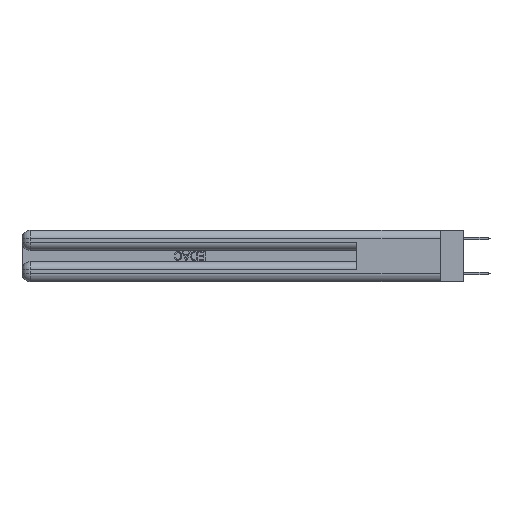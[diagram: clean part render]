
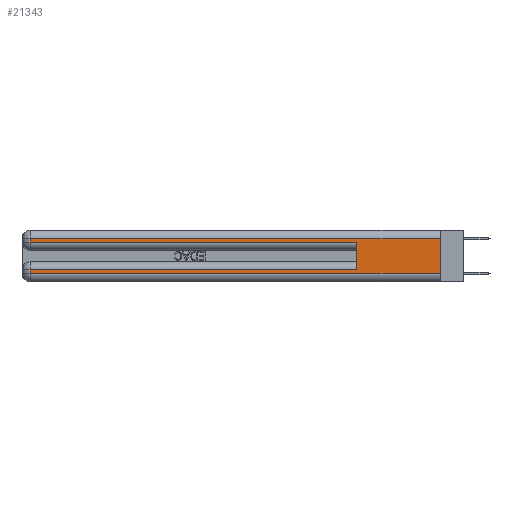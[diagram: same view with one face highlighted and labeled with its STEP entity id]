
A CAD part, left-side view. The second image highlights one B-rep face of the part: STEP entity #21343.
In plain terms, the highlighted planar face has unit normal (-1, 0, 0).
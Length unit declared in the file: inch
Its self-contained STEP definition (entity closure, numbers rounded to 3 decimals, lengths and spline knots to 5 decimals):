
#115 = CARTESIAN_POINT ( 'NONE',  ( 0., 0., 0.37 ) ) ;
#139 = VECTOR ( 'NONE', #22408, 39.37008 ) ;
#623 = ORIENTED_EDGE ( 'NONE', *, *, #24026, .T. ) ;
#768 = CARTESIAN_POINT ( 'NONE',  ( 0., 0., 0.085 ) ) ;
#996 = LINE ( 'NONE', #28972, #139 ) ;
#1272 = CARTESIAN_POINT ( 'NONE',  ( 0., 2.94, 0.31 ) ) ;
#1301 = CARTESIAN_POINT ( 'NONE',  ( 0., 0.6, 0.145 ) ) ;
#1329 = LINE ( 'NONE', #10955, #8237 ) ;
#2145 = ORIENTED_EDGE ( 'NONE', *, *, #18028, .T. ) ;
#3012 = LINE ( 'NONE', #26530, #22040 ) ;
#3297 = DIRECTION ( 'NONE',  ( 0., -1., 0. ) ) ;
#3968 = ORIENTED_EDGE ( 'NONE', *, *, #22830, .T. ) ;
#5042 = CARTESIAN_POINT ( 'NONE',  ( 0., 0., 0.31 ) ) ;
#5150 = DIRECTION ( 'NONE',  ( 1., 0., 0. ) ) ;
#6066 = VECTOR ( 'NONE', #25166, 39.37008 ) ;
#6242 = CARTESIAN_POINT ( 'NONE',  ( 0., 2.94, 0.37 ) ) ;
#6951 = ORIENTED_EDGE ( 'NONE', *, *, #24611, .F. ) ;
#7190 = VERTEX_POINT ( 'NONE', #26090 ) ;
#7719 = CARTESIAN_POINT ( 'NONE',  ( 0., 0.6, 0.285 ) ) ;
#7885 = AXIS2_PLACEMENT_3D ( 'NONE', #115, #5150, #23665 ) ;
#8119 = EDGE_CURVE ( 'NONE', #10188, #25764, #29738, .T. ) ;
#8237 = VECTOR ( 'NONE', #12975, 39.37008 ) ;
#10068 = DIRECTION ( 'NONE',  ( 0., -1., 0. ) ) ;
#10188 = VERTEX_POINT ( 'NONE', #5042 ) ;
#10955 = CARTESIAN_POINT ( 'NONE',  ( 0., 0., 0.37 ) ) ;
#11204 = VERTEX_POINT ( 'NONE', #17185 ) ;
#12676 = CARTESIAN_POINT ( 'NONE',  ( 0., 0., 0.06 ) ) ;
#12975 = DIRECTION ( 'NONE',  ( 0., 0., -1. ) ) ;
#14422 = VERTEX_POINT ( 'NONE', #7719 ) ;
#15247 = VECTOR ( 'NONE', #27297, 39.37008 ) ;
#15423 = ORIENTED_EDGE ( 'NONE', *, *, #17363, .T. ) ;
#15563 = DIRECTION ( 'NONE',  ( 0., 0., -1. ) ) ;
#15647 = EDGE_CURVE ( 'NONE', #10188, #17925, #1329, .T. ) ;
#16794 = ORIENTED_EDGE ( 'NONE', *, *, #8119, .T. ) ;
#16981 = ORIENTED_EDGE ( 'NONE', *, *, #27589, .T. ) ;
#17111 = VECTOR ( 'NONE', #15563, 39.37008 ) ;
#17115 = LINE ( 'NONE', #768, #27125 ) ;
#17185 = CARTESIAN_POINT ( 'NONE',  ( 0., 2.94, 0.285 ) ) ;
#17363 = EDGE_CURVE ( 'NONE', #25764, #11204, #27202, .T. ) ;
#17925 = VERTEX_POINT ( 'NONE', #26238 ) ;
#17942 = CARTESIAN_POINT ( 'NONE',  ( 0., 0.6, 0.085 ) ) ;
#18028 = EDGE_CURVE ( 'NONE', #11204, #14422, #3012, .T. ) ;
#19139 = CARTESIAN_POINT ( 'NONE',  ( 0., 2.94, 0.06 ) ) ;
#19998 = VERTEX_POINT ( 'NONE', #19139 ) ;
#20091 = ORIENTED_EDGE ( 'NONE', *, *, #15647, .F. ) ;
#21209 = FACE_OUTER_BOUND ( 'NONE', #24772, .T. ) ;
#21278 = DIRECTION ( 'NONE',  ( 0., 1., 0. ) ) ;
#21343 = ADVANCED_FACE ( 'NONE', ( #21209 ), #28385, .F. ) ;
#22040 = VECTOR ( 'NONE', #3297, 39.37008 ) ;
#22408 = DIRECTION ( 'NONE',  ( 0., 0., -1. ) ) ;
#22830 = EDGE_CURVE ( 'NONE', #7190, #19998, #996, .T. ) ;
#23665 = DIRECTION ( 'NONE',  ( 0., 0., -1. ) ) ;
#24026 = EDGE_CURVE ( 'NONE', #19998, #17925, #26580, .T. ) ;
#24611 = EDGE_CURVE ( 'NONE', #25688, #14422, #27288, .T. ) ;
#24772 = EDGE_LOOP ( 'NONE', ( #20091, #16794, #15423, #2145, #6951, #16981, #3968, #623 ) ) ;
#25017 = CARTESIAN_POINT ( 'NONE',  ( 0., 0., 0.31 ) ) ;
#25166 = DIRECTION ( 'NONE',  ( 0., 0., 1. ) ) ;
#25688 = VERTEX_POINT ( 'NONE', #17942 ) ;
#25764 = VERTEX_POINT ( 'NONE', #1272 ) ;
#26090 = CARTESIAN_POINT ( 'NONE',  ( 0., 2.94, 0.085 ) ) ;
#26238 = CARTESIAN_POINT ( 'NONE',  ( 0., 0., 0.06 ) ) ;
#26530 = CARTESIAN_POINT ( 'NONE',  ( 0., 0., 0.285 ) ) ;
#26580 = LINE ( 'NONE', #12676, #27538 ) ;
#27125 = VECTOR ( 'NONE', #21278, 39.37008 ) ;
#27202 = LINE ( 'NONE', #6242, #17111 ) ;
#27288 = LINE ( 'NONE', #1301, #6066 ) ;
#27297 = DIRECTION ( 'NONE',  ( 0., 1., 0. ) ) ;
#27538 = VECTOR ( 'NONE', #10068, 39.37008 ) ;
#27589 = EDGE_CURVE ( 'NONE', #25688, #7190, #17115, .T. ) ;
#28385 = PLANE ( 'NONE',  #7885 ) ;
#28972 = CARTESIAN_POINT ( 'NONE',  ( 0., 2.94, 0.37 ) ) ;
#29738 = LINE ( 'NONE', #25017, #15247 ) ;
